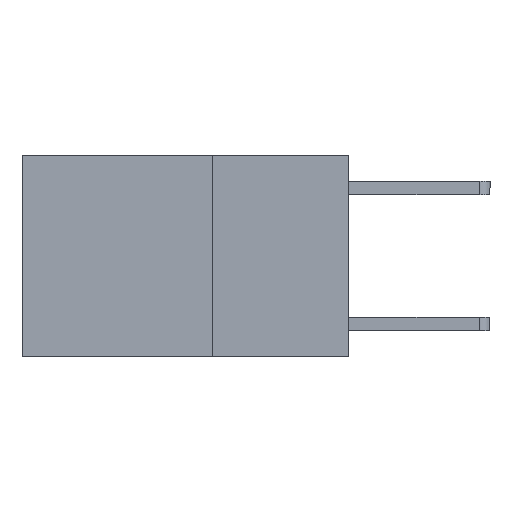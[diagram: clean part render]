
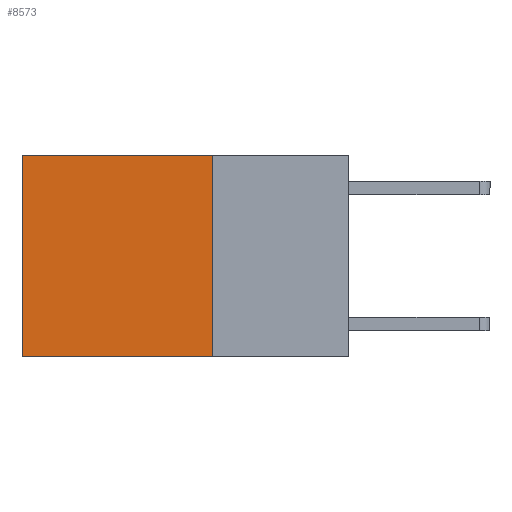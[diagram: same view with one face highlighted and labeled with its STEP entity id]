
A CAD part, left-side view. The second image highlights one B-rep face of the part: STEP entity #8573.
In plain terms, the highlighted planar face has unit normal (-1, 0, 0).
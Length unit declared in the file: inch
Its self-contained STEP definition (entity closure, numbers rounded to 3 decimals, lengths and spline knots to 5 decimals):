
#167 = VECTOR ( 'NONE', #6672, 39.37008 ) ;
#434 = CARTESIAN_POINT ( 'NONE',  ( 0.2625, 0.25, -0.37 ) ) ;
#976 = DIRECTION ( 'NONE',  ( 0., 0., -1. ) ) ;
#1096 = ORIENTED_EDGE ( 'NONE', *, *, #6997, .F. ) ;
#1681 = LINE ( 'NONE', #9338, #5126 ) ;
#3451 = ORIENTED_EDGE ( 'NONE', *, *, #8375, .F. ) ;
#3482 = FACE_OUTER_BOUND ( 'NONE', #8118, .T. ) ;
#3831 = LINE ( 'NONE', #5321, #6597 ) ;
#3989 = ORIENTED_EDGE ( 'NONE', *, *, #8406, .T. ) ;
#4205 = VECTOR ( 'NONE', #976, 39.37008 ) ;
#4604 = VERTEX_POINT ( 'NONE', #434 ) ;
#4688 = EDGE_CURVE ( 'NONE', #7687, #9312, #8512, .T. ) ;
#4746 = CARTESIAN_POINT ( 'NONE',  ( 0.2625, 0.25, 0. ) ) ;
#4989 = LINE ( 'NONE', #8393, #4205 ) ;
#5121 = ORIENTED_EDGE ( 'NONE', *, *, #4688, .T. ) ;
#5126 = VECTOR ( 'NONE', #6437, 39.37008 ) ;
#5321 = CARTESIAN_POINT ( 'NONE',  ( 0.2625, 0.6, 0. ) ) ;
#5644 = AXIS2_PLACEMENT_3D ( 'NONE', #6526, #9499, #7984 ) ;
#6437 = DIRECTION ( 'NONE',  ( 0., 1., 0. ) ) ;
#6526 = CARTESIAN_POINT ( 'NONE',  ( 0.2625, 0.25, 0. ) ) ;
#6597 = VECTOR ( 'NONE', #6882, 39.37008 ) ;
#6663 = CARTESIAN_POINT ( 'NONE',  ( 0.2625, 0.6, -0.37 ) ) ;
#6672 = DIRECTION ( 'NONE',  ( 0., 1., 0. ) ) ;
#6882 = DIRECTION ( 'NONE',  ( 0., 0., -1. ) ) ;
#6997 = EDGE_CURVE ( 'NONE', #4604, #7521, #1681, .T. ) ;
#7280 = PLANE ( 'NONE',  #5644 ) ;
#7521 = VERTEX_POINT ( 'NONE', #6663 ) ;
#7687 = VERTEX_POINT ( 'NONE', #4746 ) ;
#7765 = CARTESIAN_POINT ( 'NONE',  ( 0.2625, 0.25, 0. ) ) ;
#7984 = DIRECTION ( 'NONE',  ( 0., 0., -1. ) ) ;
#8072 = CARTESIAN_POINT ( 'NONE',  ( 0.2625, 0.6, 0. ) ) ;
#8118 = EDGE_LOOP ( 'NONE', ( #3989, #1096, #3451, #5121 ) ) ;
#8375 = EDGE_CURVE ( 'NONE', #7687, #4604, #4989, .T. ) ;
#8393 = CARTESIAN_POINT ( 'NONE',  ( 0.2625, 0.25, 0. ) ) ;
#8406 = EDGE_CURVE ( 'NONE', #9312, #7521, #3831, .T. ) ;
#8512 = LINE ( 'NONE', #7765, #167 ) ;
#8573 = ADVANCED_FACE ( 'NONE', ( #3482 ), #7280, .F. ) ;
#9312 = VERTEX_POINT ( 'NONE', #8072 ) ;
#9338 = CARTESIAN_POINT ( 'NONE',  ( 0.2625, 0.25, -0.37 ) ) ;
#9499 = DIRECTION ( 'NONE',  ( 1., 0., 0. ) ) ;
